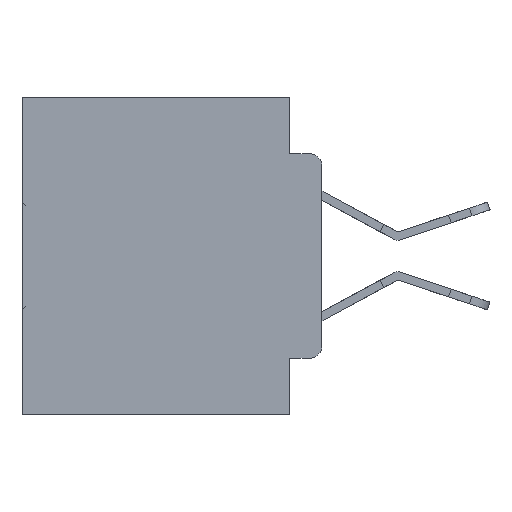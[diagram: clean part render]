
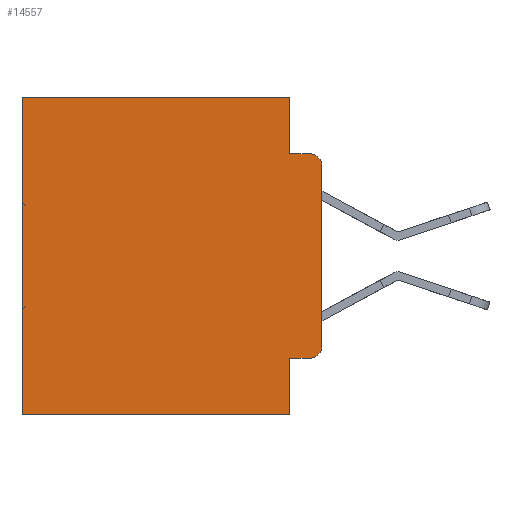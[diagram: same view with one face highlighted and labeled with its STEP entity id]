
A CAD part, left-side view. The second image highlights one B-rep face of the part: STEP entity #14557.
In plain terms, the highlighted planar face has unit normal (-1, 0, 0).
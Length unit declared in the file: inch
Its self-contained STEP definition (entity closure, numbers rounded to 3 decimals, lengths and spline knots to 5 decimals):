
#85 = CARTESIAN_POINT ( 'NONE',  ( 0.298, 0.051, -0.0885 ) ) ;
#471 = DIRECTION ( 'NONE',  ( 0., 1., 0. ) ) ;
#842 = EDGE_CURVE ( 'NONE', #11062, #4910, #27270, .T. ) ;
#885 = VECTOR ( 'NONE', #13769, 39.37008 ) ;
#2147 = CARTESIAN_POINT ( 'NONE',  ( 0.298, 0.051, -0.5 ) ) ;
#2311 = DIRECTION ( 'NONE',  ( 0., 0., -1. ) ) ;
#2626 = CARTESIAN_POINT ( 'NONE',  ( 0.298, 0.02, -0.3915 ) ) ;
#2688 = VERTEX_POINT ( 'NONE', #14793 ) ;
#2896 = CARTESIAN_POINT ( 'NONE',  ( 0.298, 0.02, -0.4115 ) ) ;
#2930 = LINE ( 'NONE', #34533, #22864 ) ;
#3711 = VERTEX_POINT ( 'NONE', #7036 ) ;
#4052 = VERTEX_POINT ( 'NONE', #2896 ) ;
#4440 = FACE_OUTER_BOUND ( 'NONE', #16239, .T. ) ;
#4910 = VERTEX_POINT ( 'NONE', #2147 ) ;
#5081 = DIRECTION ( 'NONE',  ( -1., 0., 0. ) ) ;
#5355 = DIRECTION ( 'NONE',  ( 0., 0., -1. ) ) ;
#5459 = EDGE_CURVE ( 'NONE', #32875, #3711, #24108, .T. ) ;
#5759 = VERTEX_POINT ( 'NONE', #7382 ) ;
#6167 = EDGE_CURVE ( 'NONE', #14175, #2688, #16582, .T. ) ;
#6344 = EDGE_CURVE ( 'NONE', #18449, #16028, #2930, .T. ) ;
#6553 = CARTESIAN_POINT ( 'NONE',  ( 0.298, 0., 0. ) ) ;
#7036 = CARTESIAN_POINT ( 'NONE',  ( 0.298, 0., -0.3915 ) ) ;
#7039 = EDGE_CURVE ( 'NONE', #4052, #3711, #9770, .T. ) ;
#7382 = CARTESIAN_POINT ( 'NONE',  ( 0.298, 0.02, -0.0885 ) ) ;
#8128 = VECTOR ( 'NONE', #26086, 39.37008 ) ;
#9521 = AXIS2_PLACEMENT_3D ( 'NONE', #2626, #21634, #5355 ) ;
#9770 = CIRCLE ( 'NONE', #9521, 0.02 ) ;
#10025 = CARTESIAN_POINT ( 'NONE',  ( 0.298, 0., -0.5 ) ) ;
#10060 = CARTESIAN_POINT ( 'NONE',  ( 0.298, 0.473, 0. ) ) ;
#11062 = VERTEX_POINT ( 'NONE', #29776 ) ;
#11721 = EDGE_CURVE ( 'NONE', #2688, #5759, #15488, .T. ) ;
#12001 = ORIENTED_EDGE ( 'NONE', *, *, #6167, .F. ) ;
#12942 = ORIENTED_EDGE ( 'NONE', *, *, #15390, .T. ) ;
#12944 = DIRECTION ( 'NONE',  ( 0., 0., -1. ) ) ;
#13099 = ORIENTED_EDGE ( 'NONE', *, *, #6344, .T. ) ;
#13333 = AXIS2_PLACEMENT_3D ( 'NONE', #15583, #28928, #12944 ) ;
#13454 = CARTESIAN_POINT ( 'NONE',  ( 0.298, 0.473, -0.5 ) ) ;
#13769 = DIRECTION ( 'NONE',  ( 0., -1., 0. ) ) ;
#14135 = CARTESIAN_POINT ( 'NONE',  ( 0.298, 0., 0. ) ) ;
#14175 = VERTEX_POINT ( 'NONE', #22119 ) ;
#14557 = ADVANCED_FACE ( 'NONE', ( #4440 ), #26252, .F. ) ;
#14793 = CARTESIAN_POINT ( 'NONE',  ( 0.298, 0.051, -0.0885 ) ) ;
#15302 = DIRECTION ( 'NONE',  ( 0., 0., -1. ) ) ;
#15390 = EDGE_CURVE ( 'NONE', #32875, #5759, #23037, .T. ) ;
#15442 = LINE ( 'NONE', #10025, #8128 ) ;
#15488 = LINE ( 'NONE', #85, #885 ) ;
#15583 = CARTESIAN_POINT ( 'NONE',  ( 0.298, 0., 0. ) ) ;
#16028 = VERTEX_POINT ( 'NONE', #13454 ) ;
#16239 = EDGE_LOOP ( 'NONE', ( #24835, #12942, #22202, #12001, #23898, #13099, #23121, #19980, #33481, #31396 ) ) ;
#16347 = CARTESIAN_POINT ( 'NONE',  ( 0.298, 0., -0.1085 ) ) ;
#16582 = LINE ( 'NONE', #31207, #21646 ) ;
#16716 = EDGE_CURVE ( 'NONE', #14175, #18449, #17184, .T. ) ;
#16941 = LINE ( 'NONE', #19143, #23180 ) ;
#17184 = LINE ( 'NONE', #14135, #23418 ) ;
#17704 = EDGE_CURVE ( 'NONE', #4910, #16028, #15442, .T. ) ;
#18449 = VERTEX_POINT ( 'NONE', #10060 ) ;
#19143 = CARTESIAN_POINT ( 'NONE',  ( 0.298, 0.051, -0.4115 ) ) ;
#19980 = ORIENTED_EDGE ( 'NONE', *, *, #842, .F. ) ;
#20241 = VECTOR ( 'NONE', #33291, 39.37008 ) ;
#21369 = CARTESIAN_POINT ( 'NONE',  ( 0.298, 0.02, -0.1085 ) ) ;
#21634 = DIRECTION ( 'NONE',  ( -1., 0., 0. ) ) ;
#21646 = VECTOR ( 'NONE', #15302, 39.37008 ) ;
#21810 = DIRECTION ( 'NONE',  ( 0., -1., 0. ) ) ;
#21913 = CARTESIAN_POINT ( 'NONE',  ( 0.298, 0.051, 0. ) ) ;
#22119 = CARTESIAN_POINT ( 'NONE',  ( 0.298, 0.051, 0. ) ) ;
#22202 = ORIENTED_EDGE ( 'NONE', *, *, #11721, .F. ) ;
#22864 = VECTOR ( 'NONE', #2311, 39.37008 ) ;
#23037 = CIRCLE ( 'NONE', #26312, 0.02 ) ;
#23121 = ORIENTED_EDGE ( 'NONE', *, *, #17704, .F. ) ;
#23160 = DIRECTION ( 'NONE',  ( 0., 0., -1. ) ) ;
#23180 = VECTOR ( 'NONE', #21810, 39.37008 ) ;
#23355 = EDGE_CURVE ( 'NONE', #11062, #4052, #16941, .T. ) ;
#23418 = VECTOR ( 'NONE', #471, 39.37008 ) ;
#23898 = ORIENTED_EDGE ( 'NONE', *, *, #16716, .T. ) ;
#24024 = DIRECTION ( 'NONE',  ( 0., 0., -1. ) ) ;
#24108 = LINE ( 'NONE', #6553, #30333 ) ;
#24835 = ORIENTED_EDGE ( 'NONE', *, *, #5459, .F. ) ;
#26086 = DIRECTION ( 'NONE',  ( 0., 1., 0. ) ) ;
#26252 = PLANE ( 'NONE',  #13333 ) ;
#26312 = AXIS2_PLACEMENT_3D ( 'NONE', #21369, #5081, #24024 ) ;
#27270 = LINE ( 'NONE', #21913, #20241 ) ;
#28928 = DIRECTION ( 'NONE',  ( 1., 0., 0. ) ) ;
#29776 = CARTESIAN_POINT ( 'NONE',  ( 0.298, 0.051, -0.4115 ) ) ;
#30333 = VECTOR ( 'NONE', #23160, 39.37008 ) ;
#31207 = CARTESIAN_POINT ( 'NONE',  ( 0.298, 0.051, 0. ) ) ;
#31396 = ORIENTED_EDGE ( 'NONE', *, *, #7039, .T. ) ;
#32875 = VERTEX_POINT ( 'NONE', #16347 ) ;
#33291 = DIRECTION ( 'NONE',  ( 0., 0., -1. ) ) ;
#33481 = ORIENTED_EDGE ( 'NONE', *, *, #23355, .T. ) ;
#34533 = CARTESIAN_POINT ( 'NONE',  ( 0.298, 0.473, 0. ) ) ;
